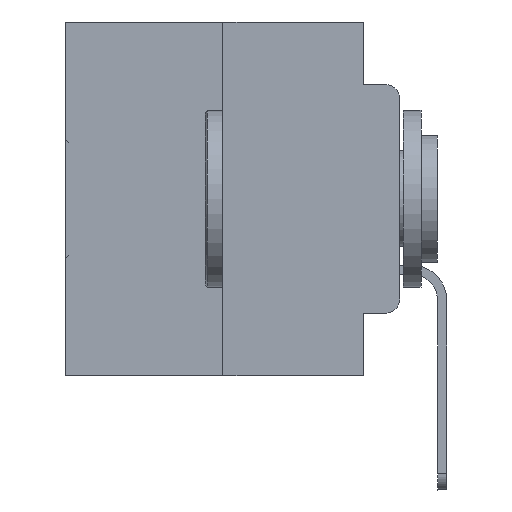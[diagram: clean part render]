
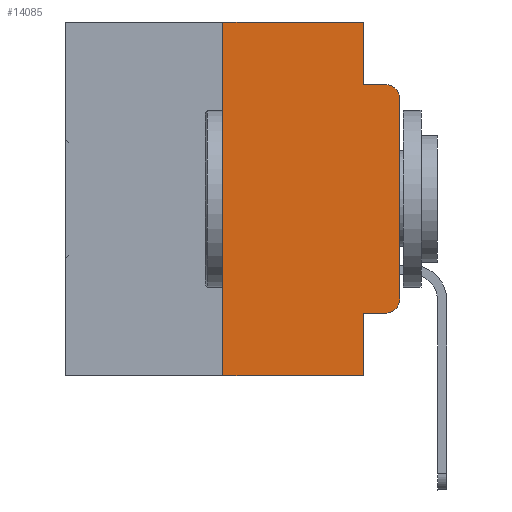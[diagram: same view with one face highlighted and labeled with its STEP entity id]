
A CAD part, left-side view. The second image highlights one B-rep face of the part: STEP entity #14085.
In plain terms, the highlighted planar face has unit normal (-1, 0, 0).
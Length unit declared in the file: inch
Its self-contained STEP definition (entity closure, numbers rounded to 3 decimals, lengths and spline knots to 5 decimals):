
#58 = DIRECTION ( 'NONE',  ( 0., -1., 0. ) ) ;
#543 = EDGE_CURVE ( 'NONE', #17679, #23805, #27505, .T. ) ;
#1580 = VECTOR ( 'NONE', #7708, 39.37008 ) ;
#1962 = DIRECTION ( 'NONE',  ( 0., 0., -1. ) ) ;
#2089 = CARTESIAN_POINT ( 'NONE',  ( 0., 0.051, -0.4115 ) ) ;
#2284 = DIRECTION ( 'NONE',  ( 0., 0., -1. ) ) ;
#2410 = CARTESIAN_POINT ( 'NONE',  ( 0., 0.25, 0. ) ) ;
#2488 = CARTESIAN_POINT ( 'NONE',  ( 0., 0., 0. ) ) ;
#2519 = VERTEX_POINT ( 'NONE', #6576 ) ;
#2581 = LINE ( 'NONE', #2410, #20847 ) ;
#2617 = EDGE_LOOP ( 'NONE', ( #6335, #5168, #28410, #28099, #9092, #6797, #9615, #24041, #19358, #6693 ) ) ;
#2928 = CARTESIAN_POINT ( 'NONE',  ( 0., 0.25, -0.5 ) ) ;
#3483 = CARTESIAN_POINT ( 'NONE',  ( 0., 0.051, -0.0885 ) ) ;
#3493 = CIRCLE ( 'NONE', #24710, 0.02 ) ;
#3985 = EDGE_CURVE ( 'NONE', #24277, #29854, #14649, .T. ) ;
#4262 = CARTESIAN_POINT ( 'NONE',  ( 0., 0.02, -0.1085 ) ) ;
#4712 = LINE ( 'NONE', #14629, #32032 ) ;
#5168 = ORIENTED_EDGE ( 'NONE', *, *, #24247, .T. ) ;
#5431 = VECTOR ( 'NONE', #18833, 39.37008 ) ;
#5853 = VERTEX_POINT ( 'NONE', #11166 ) ;
#6335 = ORIENTED_EDGE ( 'NONE', *, *, #27708, .T. ) ;
#6576 = CARTESIAN_POINT ( 'NONE',  ( 0., 0., -0.1085 ) ) ;
#6693 = ORIENTED_EDGE ( 'NONE', *, *, #543, .T. ) ;
#6797 = ORIENTED_EDGE ( 'NONE', *, *, #7495, .F. ) ;
#6896 = EDGE_CURVE ( 'NONE', #27369, #16045, #6966, .T. ) ;
#6966 = LINE ( 'NONE', #20828, #31712 ) ;
#7300 = CARTESIAN_POINT ( 'NONE',  ( 0., 0.02, -0.3915 ) ) ;
#7384 = VERTEX_POINT ( 'NONE', #2089 ) ;
#7495 = EDGE_CURVE ( 'NONE', #15877, #24277, #2581, .T. ) ;
#7708 = DIRECTION ( 'NONE',  ( 0., -1., 0. ) ) ;
#7876 = EDGE_CURVE ( 'NONE', #15877, #5853, #12272, .T. ) ;
#8062 = CARTESIAN_POINT ( 'NONE',  ( 0., 0.02, -0.4115 ) ) ;
#8493 = DIRECTION ( 'NONE',  ( 0., -1., 0. ) ) ;
#9092 = ORIENTED_EDGE ( 'NONE', *, *, #3985, .F. ) ;
#9131 = DIRECTION ( 'NONE',  ( -1., 0., 0. ) ) ;
#9421 = CARTESIAN_POINT ( 'NONE',  ( 0., 0.051, 0. ) ) ;
#9615 = ORIENTED_EDGE ( 'NONE', *, *, #7876, .T. ) ;
#9992 = CARTESIAN_POINT ( 'NONE',  ( 0., 0.473, -0.5 ) ) ;
#11166 = CARTESIAN_POINT ( 'NONE',  ( 0., 0.051, -0.5 ) ) ;
#12272 = LINE ( 'NONE', #9992, #1580 ) ;
#13530 = AXIS2_PLACEMENT_3D ( 'NONE', #7300, #14136, #1962 ) ;
#13625 = CARTESIAN_POINT ( 'NONE',  ( 0., 0., -0.3915 ) ) ;
#13666 = PLANE ( 'NONE',  #14761 ) ;
#14085 = ADVANCED_FACE ( 'NONE', ( #25974 ), #13666, .F. ) ;
#14136 = DIRECTION ( 'NONE',  ( -1., 0., 0. ) ) ;
#14629 = CARTESIAN_POINT ( 'NONE',  ( 0., 0.051, 0. ) ) ;
#14649 = LINE ( 'NONE', #31985, #30090 ) ;
#14761 = AXIS2_PLACEMENT_3D ( 'NONE', #31009, #31173, #18674 ) ;
#15877 = VERTEX_POINT ( 'NONE', #2928 ) ;
#16045 = VERTEX_POINT ( 'NONE', #18629 ) ;
#17538 = EDGE_CURVE ( 'NONE', #7384, #5853, #18992, .T. ) ;
#17563 = EDGE_CURVE ( 'NONE', #29854, #27369, #4712, .T. ) ;
#17679 = VERTEX_POINT ( 'NONE', #8062 ) ;
#18629 = CARTESIAN_POINT ( 'NONE',  ( 0., 0.02, -0.0885 ) ) ;
#18674 = DIRECTION ( 'NONE',  ( 0., 0., -1. ) ) ;
#18833 = DIRECTION ( 'NONE',  ( 0., -1., 0. ) ) ;
#18992 = LINE ( 'NONE', #9421, #20644 ) ;
#19358 = ORIENTED_EDGE ( 'NONE', *, *, #31426, .T. ) ;
#19597 = DIRECTION ( 'NONE',  ( 0., 0., 1. ) ) ;
#20644 = VECTOR ( 'NONE', #28896, 39.37008 ) ;
#20828 = CARTESIAN_POINT ( 'NONE',  ( 0., 0.051, -0.0885 ) ) ;
#20847 = VECTOR ( 'NONE', #19597, 39.37008 ) ;
#22817 = VECTOR ( 'NONE', #26973, 39.37008 ) ;
#23805 = VERTEX_POINT ( 'NONE', #13625 ) ;
#24041 = ORIENTED_EDGE ( 'NONE', *, *, #17538, .F. ) ;
#24199 = CARTESIAN_POINT ( 'NONE',  ( 0., 0.25, 0. ) ) ;
#24247 = EDGE_CURVE ( 'NONE', #2519, #16045, #3493, .T. ) ;
#24277 = VERTEX_POINT ( 'NONE', #24199 ) ;
#24710 = AXIS2_PLACEMENT_3D ( 'NONE', #4262, #9131, #28613 ) ;
#25974 = FACE_OUTER_BOUND ( 'NONE', #2617, .T. ) ;
#26128 = LINE ( 'NONE', #31179, #5431 ) ;
#26973 = DIRECTION ( 'NONE',  ( 0., 0., 1. ) ) ;
#27369 = VERTEX_POINT ( 'NONE', #3483 ) ;
#27505 = CIRCLE ( 'NONE', #13530, 0.02 ) ;
#27708 = EDGE_CURVE ( 'NONE', #23805, #2519, #29103, .T. ) ;
#28099 = ORIENTED_EDGE ( 'NONE', *, *, #17563, .F. ) ;
#28410 = ORIENTED_EDGE ( 'NONE', *, *, #6896, .F. ) ;
#28613 = DIRECTION ( 'NONE',  ( 0., 0., -1. ) ) ;
#28896 = DIRECTION ( 'NONE',  ( 0., 0., -1. ) ) ;
#29103 = LINE ( 'NONE', #2488, #22817 ) ;
#29854 = VERTEX_POINT ( 'NONE', #30594 ) ;
#30090 = VECTOR ( 'NONE', #58, 39.37008 ) ;
#30594 = CARTESIAN_POINT ( 'NONE',  ( 0., 0.051, 0. ) ) ;
#31009 = CARTESIAN_POINT ( 'NONE',  ( 0., 0.473, 0. ) ) ;
#31173 = DIRECTION ( 'NONE',  ( 1., 0., 0. ) ) ;
#31179 = CARTESIAN_POINT ( 'NONE',  ( 0., 0.051, -0.4115 ) ) ;
#31426 = EDGE_CURVE ( 'NONE', #7384, #17679, #26128, .T. ) ;
#31712 = VECTOR ( 'NONE', #8493, 39.37008 ) ;
#31985 = CARTESIAN_POINT ( 'NONE',  ( 0., 0.473, 0. ) ) ;
#32032 = VECTOR ( 'NONE', #2284, 39.37008 ) ;
